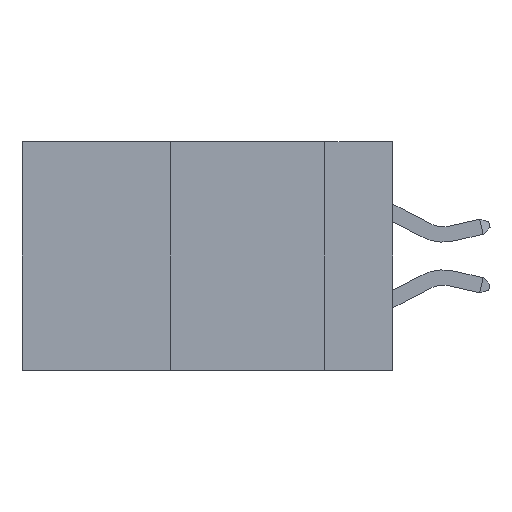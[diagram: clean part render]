
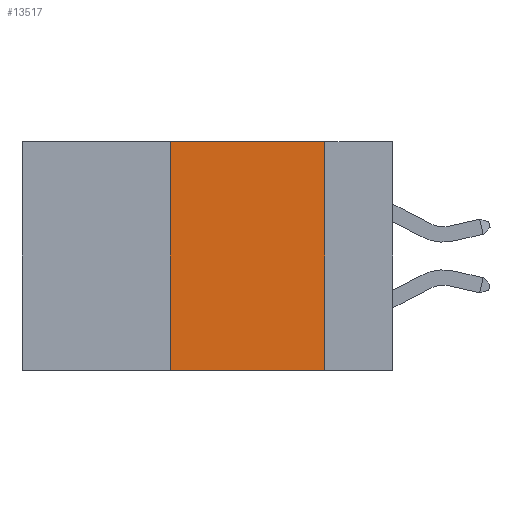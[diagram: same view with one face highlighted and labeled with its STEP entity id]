
A CAD part, left-side view. The second image highlights one B-rep face of the part: STEP entity #13517.
In plain terms, the highlighted planar face has unit normal (-1, 0, 0).
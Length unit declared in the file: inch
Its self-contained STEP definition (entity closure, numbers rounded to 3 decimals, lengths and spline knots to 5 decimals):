
#552 = VECTOR ( 'NONE', #22372, 39.37008 ) ;
#688 = ORIENTED_EDGE ( 'NONE', *, *, #43617, .T. ) ;
#2338 = CARTESIAN_POINT ( 'NONE',  ( 0., 0.36, 0. ) ) ;
#2433 = VERTEX_POINT ( 'NONE', #13490 ) ;
#2992 = LINE ( 'NONE', #2338, #31223 ) ;
#4032 = DIRECTION ( 'NONE',  ( 0., -1., 0. ) ) ;
#5882 = DIRECTION ( 'NONE',  ( 0., 0., -1. ) ) ;
#9908 = DIRECTION ( 'NONE',  ( 0., 0., 1. ) ) ;
#10526 = CARTESIAN_POINT ( 'NONE',  ( 0., 0.6, -0.37 ) ) ;
#11588 = CARTESIAN_POINT ( 'NONE',  ( 0., 0.11, -0.37 ) ) ;
#12394 = EDGE_LOOP ( 'NONE', ( #32761, #43774, #39816, #688 ) ) ;
#13225 = VERTEX_POINT ( 'NONE', #37460 ) ;
#13490 = CARTESIAN_POINT ( 'NONE',  ( 0., 0.11, 0. ) ) ;
#13517 = ADVANCED_FACE ( 'NONE', ( #29398 ), #26035, .F. ) ;
#14784 = VECTOR ( 'NONE', #31094, 39.37008 ) ;
#16158 = EDGE_CURVE ( 'NONE', #2433, #23686, #36020, .T. ) ;
#16801 = CARTESIAN_POINT ( 'NONE',  ( 0., 0.6, 0. ) ) ;
#22372 = DIRECTION ( 'NONE',  ( 0., 0., -1. ) ) ;
#23686 = VERTEX_POINT ( 'NONE', #11588 ) ;
#26035 = PLANE ( 'NONE',  #32483 ) ;
#27090 = VECTOR ( 'NONE', #4032, 39.37008 ) ;
#27540 = LINE ( 'NONE', #10526, #27090 ) ;
#29398 = FACE_OUTER_BOUND ( 'NONE', #12394, .T. ) ;
#30438 = LINE ( 'NONE', #16801, #14784 ) ;
#31094 = DIRECTION ( 'NONE',  ( 0., -1., 0. ) ) ;
#31223 = VECTOR ( 'NONE', #9908, 39.37008 ) ;
#32210 = CARTESIAN_POINT ( 'NONE',  ( 0., 0.11, 0. ) ) ;
#32483 = AXIS2_PLACEMENT_3D ( 'NONE', #42795, #39665, #5882 ) ;
#32761 = ORIENTED_EDGE ( 'NONE', *, *, #16158, .F. ) ;
#34393 = EDGE_CURVE ( 'NONE', #13225, #2433, #30438, .T. ) ;
#35850 = VERTEX_POINT ( 'NONE', #40958 ) ;
#36020 = LINE ( 'NONE', #32210, #552 ) ;
#37460 = CARTESIAN_POINT ( 'NONE',  ( 0., 0.36, 0. ) ) ;
#39665 = DIRECTION ( 'NONE',  ( 1., 0., 0. ) ) ;
#39816 = ORIENTED_EDGE ( 'NONE', *, *, #40460, .F. ) ;
#40460 = EDGE_CURVE ( 'NONE', #35850, #13225, #2992, .T. ) ;
#40958 = CARTESIAN_POINT ( 'NONE',  ( 0., 0.36, -0.37 ) ) ;
#42795 = CARTESIAN_POINT ( 'NONE',  ( 0., 0.6, 0. ) ) ;
#43617 = EDGE_CURVE ( 'NONE', #35850, #23686, #27540, .T. ) ;
#43774 = ORIENTED_EDGE ( 'NONE', *, *, #34393, .F. ) ;
